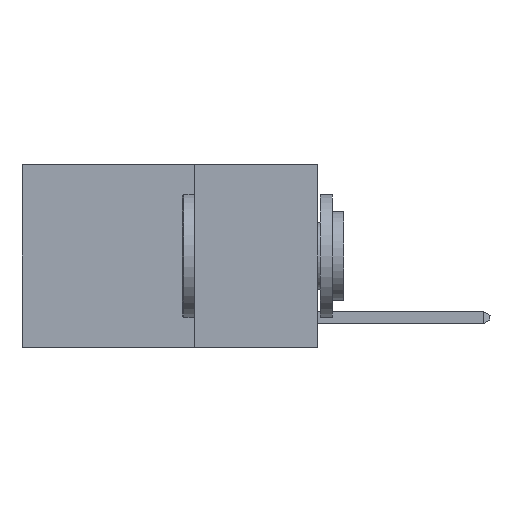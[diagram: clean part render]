
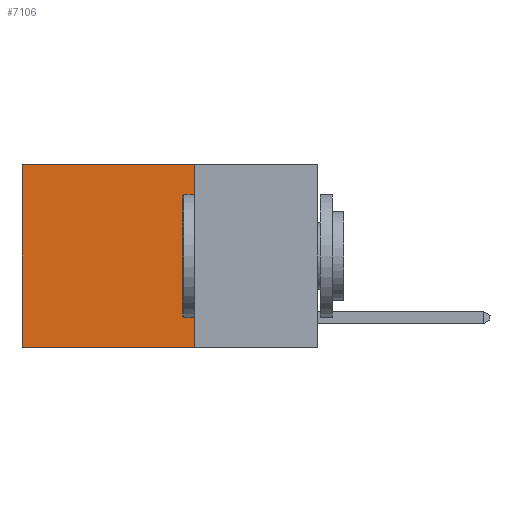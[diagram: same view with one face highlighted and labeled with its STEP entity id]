
A CAD part, left-side view. The second image highlights one B-rep face of the part: STEP entity #7106.
In plain terms, the highlighted planar face has unit normal (-1, 0, 0).
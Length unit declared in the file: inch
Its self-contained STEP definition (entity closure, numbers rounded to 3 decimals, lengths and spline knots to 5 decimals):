
#912 = DIRECTION ( 'NONE',  ( 0., 0., -1. ) ) ;
#947 = VERTEX_POINT ( 'NONE', #9194 ) ;
#1105 = VERTEX_POINT ( 'NONE', #8732 ) ;
#1400 = EDGE_CURVE ( 'NONE', #4406, #947, #7444, .T. ) ;
#1493 = CARTESIAN_POINT ( 'NONE',  ( 0.2625, 0.25, 0. ) ) ;
#1970 = VECTOR ( 'NONE', #912, 39.37008 ) ;
#2081 = CARTESIAN_POINT ( 'NONE',  ( 0.2625, 0.25, 0. ) ) ;
#2469 = LINE ( 'NONE', #5153, #10641 ) ;
#2945 = DIRECTION ( 'NONE',  ( 0., 1., 0. ) ) ;
#3301 = FACE_OUTER_BOUND ( 'NONE', #4394, .T. ) ;
#3358 = DIRECTION ( 'NONE',  ( 0., 0., -1. ) ) ;
#3382 = CARTESIAN_POINT ( 'NONE',  ( 0.2625, 0.25, 0. ) ) ;
#3488 = CARTESIAN_POINT ( 'NONE',  ( 0.2625, 0.25, 0. ) ) ;
#3625 = ORIENTED_EDGE ( 'NONE', *, *, #8909, .T. ) ;
#3775 = EDGE_CURVE ( 'NONE', #1105, #947, #2469, .T. ) ;
#4394 = EDGE_LOOP ( 'NONE', ( #7132, #7423, #4719, #3625 ) ) ;
#4406 = VERTEX_POINT ( 'NONE', #5600 ) ;
#4452 = LINE ( 'NONE', #3382, #1970 ) ;
#4719 = ORIENTED_EDGE ( 'NONE', *, *, #9766, .F. ) ;
#5153 = CARTESIAN_POINT ( 'NONE',  ( 0.2625, 0.6, 0. ) ) ;
#5482 = VECTOR ( 'NONE', #2945, 39.37008 ) ;
#5600 = CARTESIAN_POINT ( 'NONE',  ( 0.2625, 0.25, -0.37 ) ) ;
#6436 = VERTEX_POINT ( 'NONE', #3488 ) ;
#6757 = DIRECTION ( 'NONE',  ( 1., 0., 0. ) ) ;
#6920 = PLANE ( 'NONE',  #9208 ) ;
#7106 = ADVANCED_FACE ( 'NONE', ( #3301 ), #6920, .F. ) ;
#7132 = ORIENTED_EDGE ( 'NONE', *, *, #3775, .T. ) ;
#7423 = ORIENTED_EDGE ( 'NONE', *, *, #1400, .F. ) ;
#7444 = LINE ( 'NONE', #7864, #8924 ) ;
#7786 = DIRECTION ( 'NONE',  ( 0., 0., -1. ) ) ;
#7864 = CARTESIAN_POINT ( 'NONE',  ( 0.2625, 0.25, -0.37 ) ) ;
#8732 = CARTESIAN_POINT ( 'NONE',  ( 0.2625, 0.6, 0. ) ) ;
#8857 = DIRECTION ( 'NONE',  ( 0., 1., 0. ) ) ;
#8909 = EDGE_CURVE ( 'NONE', #6436, #1105, #11408, .T. ) ;
#8924 = VECTOR ( 'NONE', #8857, 39.37008 ) ;
#9194 = CARTESIAN_POINT ( 'NONE',  ( 0.2625, 0.6, -0.37 ) ) ;
#9208 = AXIS2_PLACEMENT_3D ( 'NONE', #1493, #6757, #3358 ) ;
#9766 = EDGE_CURVE ( 'NONE', #6436, #4406, #4452, .T. ) ;
#10641 = VECTOR ( 'NONE', #7786, 39.37008 ) ;
#11408 = LINE ( 'NONE', #2081, #5482 ) ;
